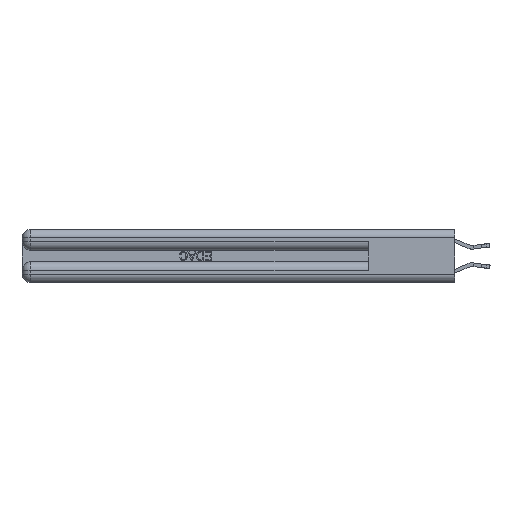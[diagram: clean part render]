
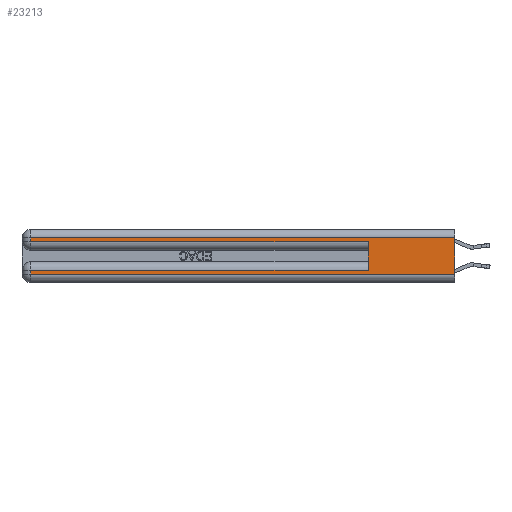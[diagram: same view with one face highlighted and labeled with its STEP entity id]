
A CAD part, left-side view. The second image highlights one B-rep face of the part: STEP entity #23213.
In plain terms, the highlighted planar face has unit normal (-1, 0, 0).
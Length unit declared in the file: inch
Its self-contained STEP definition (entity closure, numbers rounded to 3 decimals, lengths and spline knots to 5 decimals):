
#631 = LINE ( 'NONE', #2533, #14366 ) ;
#823 = LINE ( 'NONE', #13726, #10183 ) ;
#1173 = CARTESIAN_POINT ( 'NONE',  ( 0., 0., 0.06 ) ) ;
#2139 = CARTESIAN_POINT ( 'NONE',  ( 0., 0., 0.06 ) ) ;
#2304 = EDGE_CURVE ( 'NONE', #20934, #24579, #3471, .T. ) ;
#2533 = CARTESIAN_POINT ( 'NONE',  ( 0., 0., 0.31 ) ) ;
#3109 = EDGE_LOOP ( 'NONE', ( #17689, #28089, #8756, #12537, #20438, #17637, #5666, #19283 ) ) ;
#3154 = CARTESIAN_POINT ( 'NONE',  ( 0., 0., 0.285 ) ) ;
#3471 = LINE ( 'NONE', #2139, #9932 ) ;
#3602 = VERTEX_POINT ( 'NONE', #12619 ) ;
#3651 = VECTOR ( 'NONE', #24856, 39.37008 ) ;
#4158 = LINE ( 'NONE', #21816, #25482 ) ;
#4284 = CARTESIAN_POINT ( 'NONE',  ( 0., 2.94, 0.37 ) ) ;
#4528 = VECTOR ( 'NONE', #6629, 39.37008 ) ;
#5020 = LINE ( 'NONE', #3154, #19088 ) ;
#5666 = ORIENTED_EDGE ( 'NONE', *, *, #20018, .T. ) ;
#6532 = CARTESIAN_POINT ( 'NONE',  ( 0., 2.94, 0.37 ) ) ;
#6629 = DIRECTION ( 'NONE',  ( 0., 0., -1. ) ) ;
#6766 = DIRECTION ( 'NONE',  ( 0., -1., 0. ) ) ;
#6862 = DIRECTION ( 'NONE',  ( 0., 1., 0. ) ) ;
#8235 = VERTEX_POINT ( 'NONE', #26468 ) ;
#8756 = ORIENTED_EDGE ( 'NONE', *, *, #16420, .T. ) ;
#9932 = VECTOR ( 'NONE', #6766, 39.37008 ) ;
#9955 = EDGE_CURVE ( 'NONE', #15993, #19939, #20944, .T. ) ;
#10154 = CARTESIAN_POINT ( 'NONE',  ( 0., 2.94, 0.06 ) ) ;
#10183 = VECTOR ( 'NONE', #18446, 39.37008 ) ;
#10484 = LINE ( 'NONE', #4284, #3651 ) ;
#10639 = VERTEX_POINT ( 'NONE', #12606 ) ;
#11435 = VERTEX_POINT ( 'NONE', #23977 ) ;
#12018 = DIRECTION ( 'NONE',  ( 0., -1., 0. ) ) ;
#12239 = PLANE ( 'NONE',  #24547 ) ;
#12537 = ORIENTED_EDGE ( 'NONE', *, *, #29391, .T. ) ;
#12606 = CARTESIAN_POINT ( 'NONE',  ( 0., 2.94, 0.285 ) ) ;
#12619 = CARTESIAN_POINT ( 'NONE',  ( 0., 2.94, 0.31 ) ) ;
#12800 = DIRECTION ( 'NONE',  ( 0., 0., 1. ) ) ;
#13726 = CARTESIAN_POINT ( 'NONE',  ( 0., 0., 0.37 ) ) ;
#14366 = VECTOR ( 'NONE', #26041, 39.37008 ) ;
#14571 = DIRECTION ( 'NONE',  ( 1., 0., 0. ) ) ;
#14827 = VECTOR ( 'NONE', #6862, 39.37008 ) ;
#15241 = EDGE_CURVE ( 'NONE', #11435, #3602, #631, .T. ) ;
#15806 = CARTESIAN_POINT ( 'NONE',  ( 0., 2.94, 0.085 ) ) ;
#15993 = VERTEX_POINT ( 'NONE', #25370 ) ;
#16420 = EDGE_CURVE ( 'NONE', #3602, #10639, #29790, .T. ) ;
#16896 = DIRECTION ( 'NONE',  ( 0., 0., -1. ) ) ;
#17637 = ORIENTED_EDGE ( 'NONE', *, *, #9955, .T. ) ;
#17689 = ORIENTED_EDGE ( 'NONE', *, *, #17824, .F. ) ;
#17824 = EDGE_CURVE ( 'NONE', #11435, #24579, #823, .T. ) ;
#18446 = DIRECTION ( 'NONE',  ( 0., 0., -1. ) ) ;
#19088 = VECTOR ( 'NONE', #12018, 39.37008 ) ;
#19283 = ORIENTED_EDGE ( 'NONE', *, *, #2304, .T. ) ;
#19939 = VERTEX_POINT ( 'NONE', #15806 ) ;
#20018 = EDGE_CURVE ( 'NONE', #19939, #20934, #10484, .T. ) ;
#20438 = ORIENTED_EDGE ( 'NONE', *, *, #26767, .F. ) ;
#20934 = VERTEX_POINT ( 'NONE', #10154 ) ;
#20944 = LINE ( 'NONE', #27659, #14827 ) ;
#21816 = CARTESIAN_POINT ( 'NONE',  ( 0., 0.6, 0.145 ) ) ;
#23213 = ADVANCED_FACE ( 'NONE', ( #28908 ), #12239, .F. ) ;
#23977 = CARTESIAN_POINT ( 'NONE',  ( 0., 0., 0.31 ) ) ;
#24547 = AXIS2_PLACEMENT_3D ( 'NONE', #28406, #14571, #16896 ) ;
#24579 = VERTEX_POINT ( 'NONE', #1173 ) ;
#24856 = DIRECTION ( 'NONE',  ( 0., 0., -1. ) ) ;
#25370 = CARTESIAN_POINT ( 'NONE',  ( 0., 0.6, 0.085 ) ) ;
#25482 = VECTOR ( 'NONE', #12800, 39.37008 ) ;
#26041 = DIRECTION ( 'NONE',  ( 0., 1., 0. ) ) ;
#26468 = CARTESIAN_POINT ( 'NONE',  ( 0., 0.6, 0.285 ) ) ;
#26767 = EDGE_CURVE ( 'NONE', #15993, #8235, #4158, .T. ) ;
#27659 = CARTESIAN_POINT ( 'NONE',  ( 0., 0., 0.085 ) ) ;
#28089 = ORIENTED_EDGE ( 'NONE', *, *, #15241, .T. ) ;
#28406 = CARTESIAN_POINT ( 'NONE',  ( 0., 0., 0.37 ) ) ;
#28908 = FACE_OUTER_BOUND ( 'NONE', #3109, .T. ) ;
#29391 = EDGE_CURVE ( 'NONE', #10639, #8235, #5020, .T. ) ;
#29790 = LINE ( 'NONE', #6532, #4528 ) ;
